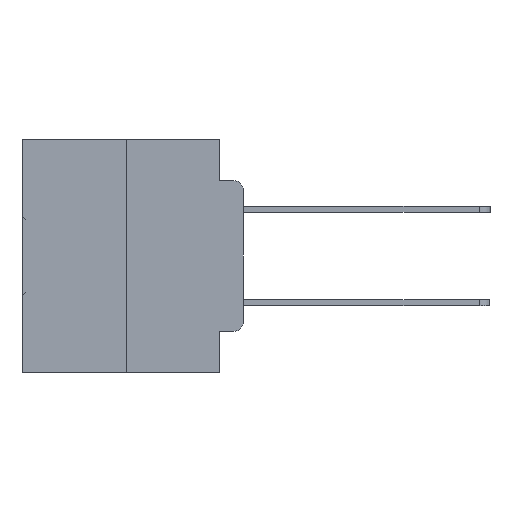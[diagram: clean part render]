
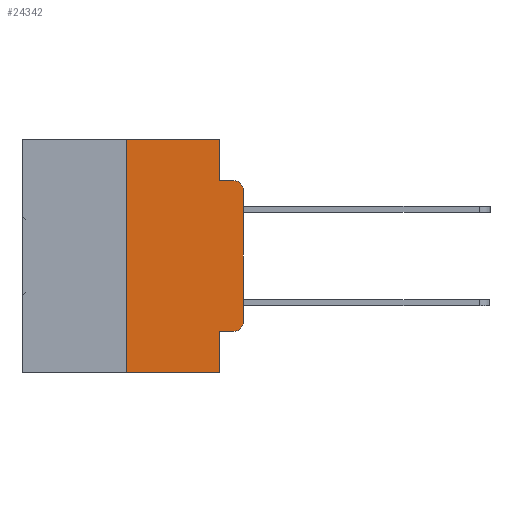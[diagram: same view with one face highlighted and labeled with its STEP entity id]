
A CAD part, left-side view. The second image highlights one B-rep face of the part: STEP entity #24342.
In plain terms, the highlighted planar face has unit normal (-1, 0, 0).
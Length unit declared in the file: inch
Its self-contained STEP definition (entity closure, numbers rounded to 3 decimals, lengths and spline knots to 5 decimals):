
#854 = ORIENTED_EDGE ( 'NONE', *, *, #25483, .T. ) ;
#1128 = DIRECTION ( 'NONE',  ( -1., 0., 0. ) ) ;
#2234 = VERTEX_POINT ( 'NONE', #12858 ) ;
#2263 = CARTESIAN_POINT ( 'NONE',  ( 0., 0., 0. ) ) ;
#2831 = VERTEX_POINT ( 'NONE', #30676 ) ;
#2887 = VECTOR ( 'NONE', #3683, 39.37008 ) ;
#2960 = CARTESIAN_POINT ( 'NONE',  ( 0., 0.02, -0.0885 ) ) ;
#3022 = EDGE_CURVE ( 'NONE', #18813, #17608, #4262, .T. ) ;
#3683 = DIRECTION ( 'NONE',  ( 0., 0., -1. ) ) ;
#4170 = CARTESIAN_POINT ( 'NONE',  ( 0., 0.02, -0.4115 ) ) ;
#4262 = LINE ( 'NONE', #18613, #24026 ) ;
#4426 = VERTEX_POINT ( 'NONE', #2960 ) ;
#4446 = CARTESIAN_POINT ( 'NONE',  ( 0., 0.051, -0.4115 ) ) ;
#5359 = LINE ( 'NONE', #13611, #18416 ) ;
#5619 = ORIENTED_EDGE ( 'NONE', *, *, #27379, .T. ) ;
#5757 = CARTESIAN_POINT ( 'NONE',  ( 0., 0.473, 0. ) ) ;
#6148 = CIRCLE ( 'NONE', #31269, 0.02 ) ;
#6909 = LINE ( 'NONE', #30495, #12173 ) ;
#7249 = CIRCLE ( 'NONE', #13277, 0.02 ) ;
#7259 = EDGE_LOOP ( 'NONE', ( #7649, #5619, #23423, #18128, #21934, #30518, #26341, #20111, #18257, #854 ) ) ;
#7345 = LINE ( 'NONE', #19305, #11823 ) ;
#7602 = VERTEX_POINT ( 'NONE', #31901 ) ;
#7649 = ORIENTED_EDGE ( 'NONE', *, *, #13065, .T. ) ;
#8426 = DIRECTION ( 'NONE',  ( 0., 0., -1. ) ) ;
#10326 = EDGE_CURVE ( 'NONE', #2234, #2831, #6909, .T. ) ;
#10822 = VECTOR ( 'NONE', #15301, 39.37008 ) ;
#11733 = CARTESIAN_POINT ( 'NONE',  ( 0., 0.02, -0.1085 ) ) ;
#11823 = VECTOR ( 'NONE', #21831, 39.37008 ) ;
#12173 = VECTOR ( 'NONE', #12729, 39.37008 ) ;
#12211 = CARTESIAN_POINT ( 'NONE',  ( 0., 0.051, -0.0885 ) ) ;
#12276 = LINE ( 'NONE', #32187, #25079 ) ;
#12729 = DIRECTION ( 'NONE',  ( 0., -1., 0. ) ) ;
#12858 = CARTESIAN_POINT ( 'NONE',  ( 0., 0.25, 0. ) ) ;
#13065 = EDGE_CURVE ( 'NONE', #14978, #15485, #26004, .T. ) ;
#13277 = AXIS2_PLACEMENT_3D ( 'NONE', #11733, #29527, #14366 ) ;
#13611 = CARTESIAN_POINT ( 'NONE',  ( 0., 0.473, -0.5 ) ) ;
#14366 = DIRECTION ( 'NONE',  ( 0., 0., -1. ) ) ;
#14862 = DIRECTION ( 'NONE',  ( 0., -1., 0. ) ) ;
#14893 = EDGE_CURVE ( 'NONE', #7602, #28878, #5359, .T. ) ;
#14978 = VERTEX_POINT ( 'NONE', #19080 ) ;
#15301 = DIRECTION ( 'NONE',  ( 0., 0., 1. ) ) ;
#15485 = VERTEX_POINT ( 'NONE', #15872 ) ;
#15872 = CARTESIAN_POINT ( 'NONE',  ( 0., 0., -0.1085 ) ) ;
#16756 = CARTESIAN_POINT ( 'NONE',  ( 0., 0.02, -0.3915 ) ) ;
#17608 = VERTEX_POINT ( 'NONE', #4170 ) ;
#18128 = ORIENTED_EDGE ( 'NONE', *, *, #20650, .F. ) ;
#18257 = ORIENTED_EDGE ( 'NONE', *, *, #3022, .T. ) ;
#18284 = VERTEX_POINT ( 'NONE', #19946 ) ;
#18304 = EDGE_CURVE ( 'NONE', #18284, #4426, #21729, .T. ) ;
#18416 = VECTOR ( 'NONE', #31322, 39.37008 ) ;
#18613 = CARTESIAN_POINT ( 'NONE',  ( 0., 0.051, -0.4115 ) ) ;
#18813 = VERTEX_POINT ( 'NONE', #4446 ) ;
#19080 = CARTESIAN_POINT ( 'NONE',  ( 0., 0., -0.3915 ) ) ;
#19305 = CARTESIAN_POINT ( 'NONE',  ( 0., 0.25, 0. ) ) ;
#19348 = DIRECTION ( 'NONE',  ( 0., 0., -1. ) ) ;
#19946 = CARTESIAN_POINT ( 'NONE',  ( 0., 0.051, -0.0885 ) ) ;
#20111 = ORIENTED_EDGE ( 'NONE', *, *, #25057, .F. ) ;
#20650 = EDGE_CURVE ( 'NONE', #2831, #18284, #12276, .T. ) ;
#21229 = FACE_OUTER_BOUND ( 'NONE', #7259, .T. ) ;
#21729 = LINE ( 'NONE', #12211, #27600 ) ;
#21831 = DIRECTION ( 'NONE',  ( 0., 0., 1. ) ) ;
#21934 = ORIENTED_EDGE ( 'NONE', *, *, #10326, .F. ) ;
#23423 = ORIENTED_EDGE ( 'NONE', *, *, #18304, .F. ) ;
#23810 = DIRECTION ( 'NONE',  ( 1., 0., 0. ) ) ;
#24026 = VECTOR ( 'NONE', #28938, 39.37008 ) ;
#24342 = ADVANCED_FACE ( 'NONE', ( #21229 ), #26213, .F. ) ;
#24686 = DIRECTION ( 'NONE',  ( 0., 0., -1. ) ) ;
#25057 = EDGE_CURVE ( 'NONE', #18813, #28878, #29401, .T. ) ;
#25079 = VECTOR ( 'NONE', #24686, 39.37008 ) ;
#25483 = EDGE_CURVE ( 'NONE', #17608, #14978, #6148, .T. ) ;
#26004 = LINE ( 'NONE', #2263, #10822 ) ;
#26104 = EDGE_CURVE ( 'NONE', #7602, #2234, #7345, .T. ) ;
#26213 = PLANE ( 'NONE',  #26453 ) ;
#26341 = ORIENTED_EDGE ( 'NONE', *, *, #14893, .T. ) ;
#26453 = AXIS2_PLACEMENT_3D ( 'NONE', #5757, #23810, #8426 ) ;
#27379 = EDGE_CURVE ( 'NONE', #15485, #4426, #7249, .T. ) ;
#27600 = VECTOR ( 'NONE', #14862, 39.37008 ) ;
#28878 = VERTEX_POINT ( 'NONE', #30724 ) ;
#28938 = DIRECTION ( 'NONE',  ( 0., -1., 0. ) ) ;
#29260 = CARTESIAN_POINT ( 'NONE',  ( 0., 0.051, 0. ) ) ;
#29401 = LINE ( 'NONE', #29260, #2887 ) ;
#29527 = DIRECTION ( 'NONE',  ( -1., 0., 0. ) ) ;
#30495 = CARTESIAN_POINT ( 'NONE',  ( 0., 0.473, 0. ) ) ;
#30518 = ORIENTED_EDGE ( 'NONE', *, *, #26104, .F. ) ;
#30676 = CARTESIAN_POINT ( 'NONE',  ( 0., 0.051, 0. ) ) ;
#30724 = CARTESIAN_POINT ( 'NONE',  ( 0., 0.051, -0.5 ) ) ;
#31269 = AXIS2_PLACEMENT_3D ( 'NONE', #16756, #1128, #19348 ) ;
#31322 = DIRECTION ( 'NONE',  ( 0., -1., 0. ) ) ;
#31901 = CARTESIAN_POINT ( 'NONE',  ( 0., 0.25, -0.5 ) ) ;
#32187 = CARTESIAN_POINT ( 'NONE',  ( 0., 0.051, 0. ) ) ;
